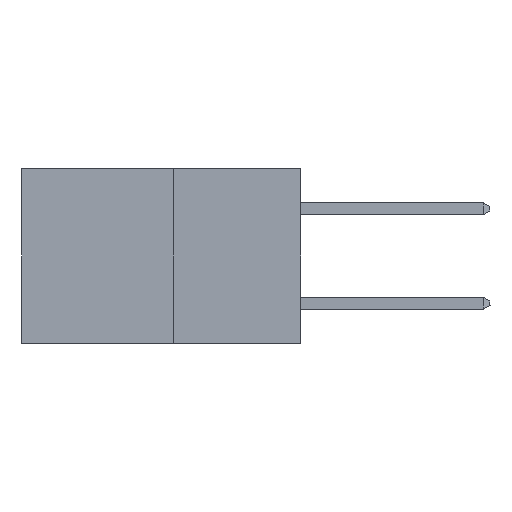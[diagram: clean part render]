
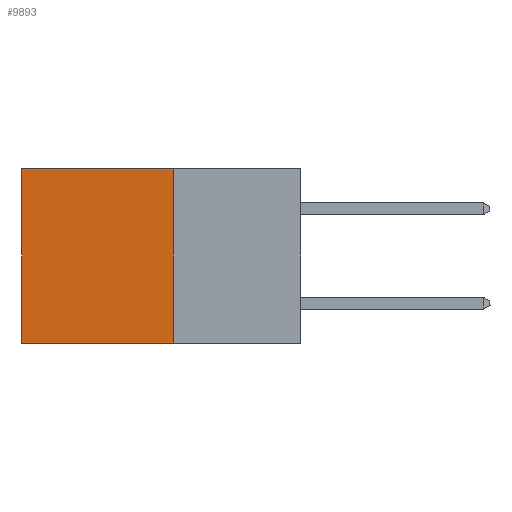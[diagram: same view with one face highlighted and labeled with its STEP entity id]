
A CAD part, left-side view. The second image highlights one B-rep face of the part: STEP entity #9893.
In plain terms, the highlighted planar face has unit normal (-1, 0, 0).
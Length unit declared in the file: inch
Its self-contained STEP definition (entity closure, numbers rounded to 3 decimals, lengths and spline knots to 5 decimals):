
#95 = ORIENTED_EDGE ( 'NONE', *, *, #7330, .T. ) ;
#676 = EDGE_LOOP ( 'NONE', ( #1554, #7791, #10605, #95 ) ) ;
#1146 = CARTESIAN_POINT ( 'NONE',  ( 0.277, 0.59, -0.37 ) ) ;
#1280 = VERTEX_POINT ( 'NONE', #10232 ) ;
#1545 = CARTESIAN_POINT ( 'NONE',  ( 0.277, 0.27, -0.37 ) ) ;
#1554 = ORIENTED_EDGE ( 'NONE', *, *, #13453, .T. ) ;
#2231 = LINE ( 'NONE', #15440, #15430 ) ;
#2691 = VECTOR ( 'NONE', #9549, 39.37008 ) ;
#2764 = LINE ( 'NONE', #1545, #15545 ) ;
#3828 = LINE ( 'NONE', #1146, #7721 ) ;
#4938 = CARTESIAN_POINT ( 'NONE',  ( 0.277, 0.59, -0.37 ) ) ;
#5018 = AXIS2_PLACEMENT_3D ( 'NONE', #5925, #5760, #5723 ) ;
#5723 = DIRECTION ( 'NONE',  ( 0., 0., -1. ) ) ;
#5760 = DIRECTION ( 'NONE',  ( 1., 0., 0. ) ) ;
#5925 = CARTESIAN_POINT ( 'NONE',  ( 0.277, 0.27, -0.37 ) ) ;
#5944 = PLANE ( 'NONE',  #5018 ) ;
#6314 = FACE_OUTER_BOUND ( 'NONE', #676, .T. ) ;
#6476 = CARTESIAN_POINT ( 'NONE',  ( 0.277, 0.27, 0. ) ) ;
#7330 = EDGE_CURVE ( 'NONE', #7351, #1280, #13324, .T. ) ;
#7351 = VERTEX_POINT ( 'NONE', #6476 ) ;
#7721 = VECTOR ( 'NONE', #13992, 39.37008 ) ;
#7791 = ORIENTED_EDGE ( 'NONE', *, *, #12215, .F. ) ;
#9549 = DIRECTION ( 'NONE',  ( 0., 1., 0. ) ) ;
#9893 = ADVANCED_FACE ( 'NONE', ( #6314 ), #5944, .F. ) ;
#10232 = CARTESIAN_POINT ( 'NONE',  ( 0.277, 0.59, 0. ) ) ;
#10605 = ORIENTED_EDGE ( 'NONE', *, *, #14645, .F. ) ;
#10650 = DIRECTION ( 'NONE',  ( 0., 0., -1. ) ) ;
#11715 = DIRECTION ( 'NONE',  ( 0., 1., 0. ) ) ;
#12215 = EDGE_CURVE ( 'NONE', #15906, #13681, #2231, .T. ) ;
#13324 = LINE ( 'NONE', #16262, #2691 ) ;
#13453 = EDGE_CURVE ( 'NONE', #1280, #13681, #3828, .T. ) ;
#13681 = VERTEX_POINT ( 'NONE', #4938 ) ;
#13992 = DIRECTION ( 'NONE',  ( 0., 0., -1. ) ) ;
#14645 = EDGE_CURVE ( 'NONE', #7351, #15906, #2764, .T. ) ;
#15430 = VECTOR ( 'NONE', #11715, 39.37008 ) ;
#15440 = CARTESIAN_POINT ( 'NONE',  ( 0.277, 0.27, -0.37 ) ) ;
#15541 = CARTESIAN_POINT ( 'NONE',  ( 0.277, 0.27, -0.37 ) ) ;
#15545 = VECTOR ( 'NONE', #10650, 39.37008 ) ;
#15906 = VERTEX_POINT ( 'NONE', #15541 ) ;
#16262 = CARTESIAN_POINT ( 'NONE',  ( 0.277, 0.27, 0. ) ) ;
